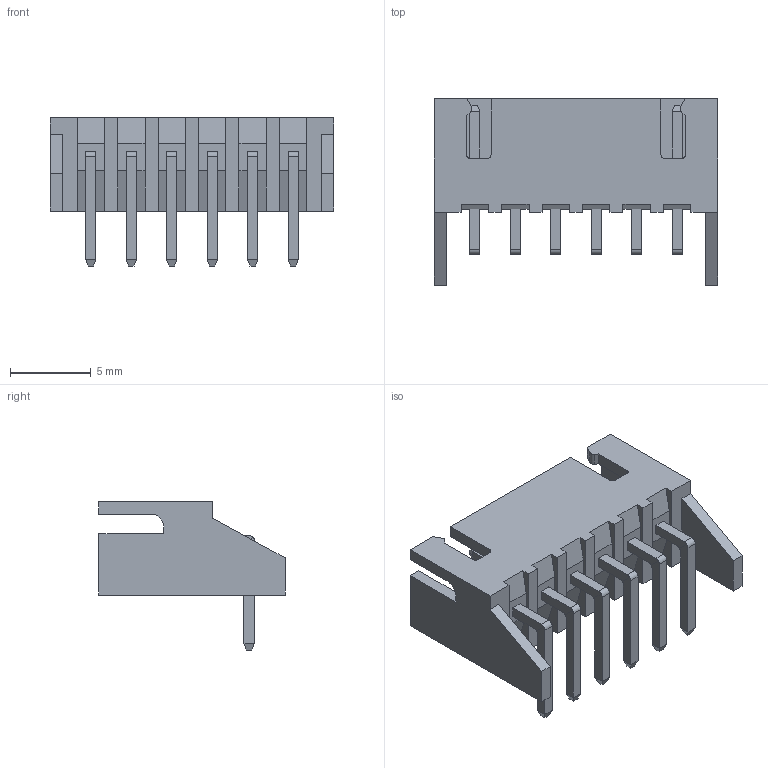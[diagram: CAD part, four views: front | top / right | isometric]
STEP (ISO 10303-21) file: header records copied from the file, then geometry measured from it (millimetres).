
FILE_DESCRIPTION (( 'STEP AP203' ), '1' );
FILE_NAME ('14K-506-416-AD1.STEP', '2024-02-22T15:43:14', ( '' ), ( '' ), 'SwSTEP 2.0', 'SolidWorks 2023', '' );
FILE_SCHEMA (( 'CONFIG_CONTROL_DESIGN' ));
Length unit declared in the file: millimetre
Products named in the file (3): 14K Series Pin with Stabilizer_16; 14K Series Pin Header Insulator with Stabilizer_506; 14K-506-416-AD1
Assembly tree (7 placements, depth 2):
  14K-506-416-AD1
    14K Series Pin Header Insulator with Stabilizer_506
    14K Series Pin with Stabilizer_16  x6
Bounding box: 17.5 x 11.5 x 9.15 mm (x, y, z)
Volume: 370.5 mm3; surface area: 1070.3 mm2
Topology: 7 solids, 7 shells, 238 faces, 624 edges, 400 vertices
Faces by surface type: plane 217, cylinder 21
Entity records: 4579 total; most frequent: CARTESIAN_POINT 742, ORIENTED_EDGE 728, DIRECTION 666, EDGE_CURVE 364, LINE 338, VECTOR 338, VERTEX_POINT 240, AXIS2_PLACEMENT_3D 164
